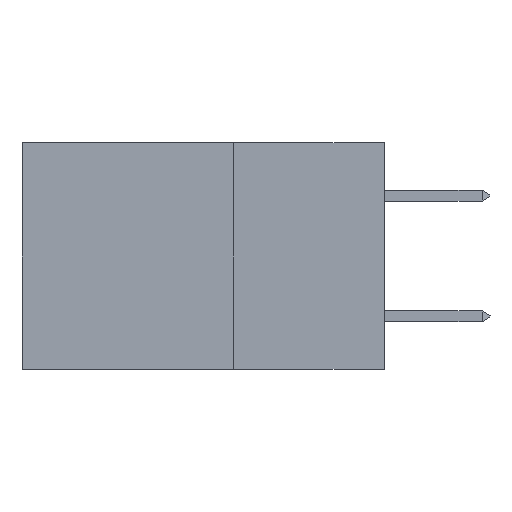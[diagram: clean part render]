
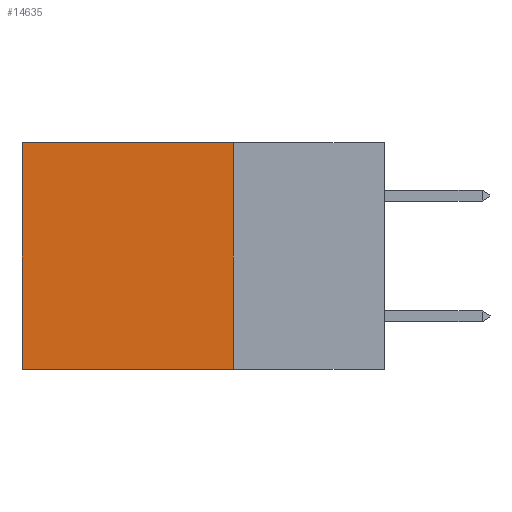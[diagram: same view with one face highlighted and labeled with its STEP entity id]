
A CAD part, left-side view. The second image highlights one B-rep face of the part: STEP entity #14635.
In plain terms, the highlighted planar face has unit normal (-1, 0, 0).
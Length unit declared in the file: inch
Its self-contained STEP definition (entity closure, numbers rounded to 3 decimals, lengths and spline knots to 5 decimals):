
#504 = EDGE_LOOP ( 'NONE', ( #584, #6513, #10559, #17569 ) ) ;
#584 = ORIENTED_EDGE ( 'NONE', *, *, #9910, .T. ) ;
#816 = VERTEX_POINT ( 'NONE', #5978 ) ;
#2275 = VECTOR ( 'NONE', #6725, 39.37008 ) ;
#2530 = VECTOR ( 'NONE', #3340, 39.37008 ) ;
#2685 = CARTESIAN_POINT ( 'NONE',  ( 0.2875, 0.6, -0.375 ) ) ;
#2800 = LINE ( 'NONE', #11342, #4873 ) ;
#3340 = DIRECTION ( 'NONE',  ( 0., 0., -1. ) ) ;
#4785 = LINE ( 'NONE', #15533, #2275 ) ;
#4873 = VECTOR ( 'NONE', #17148, 39.37008 ) ;
#5721 = VERTEX_POINT ( 'NONE', #2685 ) ;
#5746 = LINE ( 'NONE', #7228, #2530 ) ;
#5943 = FACE_OUTER_BOUND ( 'NONE', #504, .T. ) ;
#5978 = CARTESIAN_POINT ( 'NONE',  ( 0.2875, 0.6, 0. ) ) ;
#6513 = ORIENTED_EDGE ( 'NONE', *, *, #17851, .F. ) ;
#6725 = DIRECTION ( 'NONE',  ( 0., 1., 0. ) ) ;
#7228 = CARTESIAN_POINT ( 'NONE',  ( 0.2875, 0.6, -0.375 ) ) ;
#7449 = CARTESIAN_POINT ( 'NONE',  ( 0.2875, 0.25, -0.375 ) ) ;
#7811 = VERTEX_POINT ( 'NONE', #16086 ) ;
#8225 = CARTESIAN_POINT ( 'NONE',  ( 0.2875, 0.25, -0.375 ) ) ;
#8350 = DIRECTION ( 'NONE',  ( 0., 0., -1. ) ) ;
#9910 = EDGE_CURVE ( 'NONE', #816, #5721, #5746, .T. ) ;
#10178 = CARTESIAN_POINT ( 'NONE',  ( 0.2875, 0.25, 0. ) ) ;
#10559 = ORIENTED_EDGE ( 'NONE', *, *, #13087, .F. ) ;
#11098 = VECTOR ( 'NONE', #13114, 39.37008 ) ;
#11315 = EDGE_CURVE ( 'NONE', #15803, #816, #4785, .T. ) ;
#11342 = CARTESIAN_POINT ( 'NONE',  ( 0.2875, 0.25, -0.375 ) ) ;
#12494 = DIRECTION ( 'NONE',  ( 1., 0., 0. ) ) ;
#13087 = EDGE_CURVE ( 'NONE', #15803, #7811, #2800, .T. ) ;
#13114 = DIRECTION ( 'NONE',  ( 0., 1., 0. ) ) ;
#14312 = LINE ( 'NONE', #7449, #11098 ) ;
#14635 = ADVANCED_FACE ( 'NONE', ( #5943 ), #17136, .F. ) ;
#15533 = CARTESIAN_POINT ( 'NONE',  ( 0.2875, 0.25, 0. ) ) ;
#15803 = VERTEX_POINT ( 'NONE', #10178 ) ;
#16086 = CARTESIAN_POINT ( 'NONE',  ( 0.2875, 0.25, -0.375 ) ) ;
#16687 = AXIS2_PLACEMENT_3D ( 'NONE', #8225, #12494, #8350 ) ;
#17136 = PLANE ( 'NONE',  #16687 ) ;
#17148 = DIRECTION ( 'NONE',  ( 0., 0., -1. ) ) ;
#17569 = ORIENTED_EDGE ( 'NONE', *, *, #11315, .T. ) ;
#17851 = EDGE_CURVE ( 'NONE', #7811, #5721, #14312, .T. ) ;
